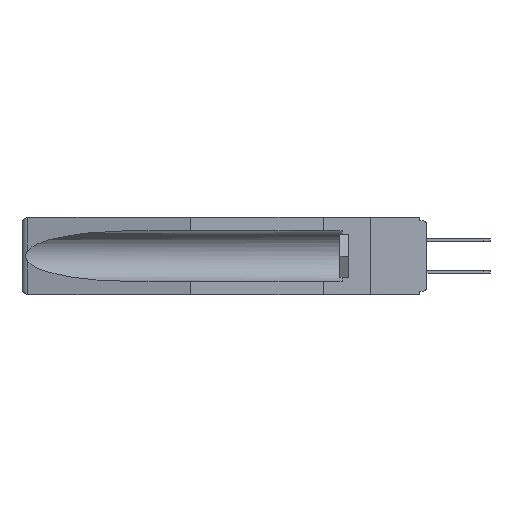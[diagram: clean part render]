
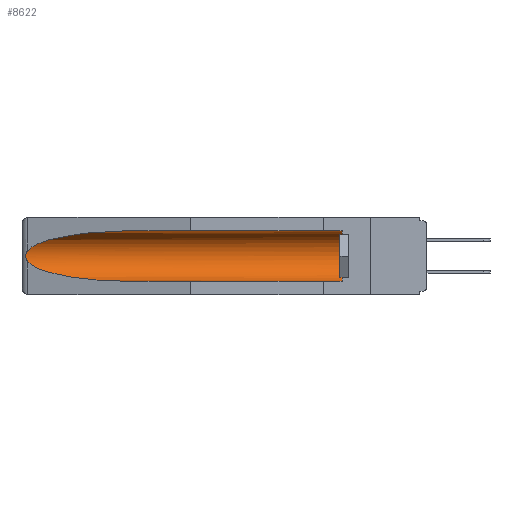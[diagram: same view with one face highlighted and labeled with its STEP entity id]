
A CAD part, left-side view. The second image highlights one B-rep face of the part: STEP entity #8622.
In plain terms, the highlighted cylindrical face has radius 2.857 mm (diameter 5.715 mm), a partial arc.
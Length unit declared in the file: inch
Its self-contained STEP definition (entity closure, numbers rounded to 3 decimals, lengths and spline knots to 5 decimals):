
#264 = CARTESIAN_POINT ( 'NONE',  ( 0.26537, 1.52718, -0.19328 ) ) ;
#686 = CARTESIAN_POINT ( 'NONE',  ( 0.155, 1.07973, -0.059 ) ) ;
#1372 = VECTOR ( 'NONE', #3937, 39.37008 ) ;
#1509 = CARTESIAN_POINT ( 'NONE',  ( 0.26654, 1.53092, -0.15636 ) ) ;
#1808 = DIRECTION ( 'NONE',  ( 0., -1., 0. ) ) ;
#2744 = CARTESIAN_POINT ( 'NONE',  ( 0.21114, 1.30732, -0.059 ) ) ;
#3155 = CARTESIAN_POINT ( 'NONE',  ( 0.155, 0.126, -0.284 ) ) ;
#3727 = B_SPLINE_CURVE_WITH_KNOTS ( 'NONE', 3,
 ( #22746, #17773, #1509, #5532, #17923, #7298, #10869, #16222, #19556, #264 ),
 .UNSPECIFIED., .F., .F.,
 ( 4, 2, 2, 2, 4 ),
 ( 0., 0.00029, 0.00058, 0.00087, 0.00117 ),
 .UNSPECIFIED. ) ;
#3937 = DIRECTION ( 'NONE',  ( 0., 1., 0. ) ) ;
#4163 = LINE ( 'NONE', #5238, #1372 ) ;
#4314 = CARTESIAN_POINT ( 'NONE',  ( 0.26537, 1.52718, -0.19328 ) ) ;
#5137 = VERTEX_POINT ( 'NONE', #3155 ) ;
#5238 = CARTESIAN_POINT ( 'NONE',  ( 0.155, -0.30754, -0.059 ) ) ;
#5261 = CYLINDRICAL_SURFACE ( 'NONE', #6894, 0.1125 ) ;
#5532 = CARTESIAN_POINT ( 'NONE',  ( 0.2673, 1.5327, -0.16383 ) ) ;
#5998 = EDGE_CURVE ( 'NONE', #5137, #9668, #10401, .T. ) ;
#6894 = AXIS2_PLACEMENT_3D ( 'NONE', #11008, #7442, #7355 ) ;
#7261 = EDGE_CURVE ( 'NONE', #18833, #18517, #3727, .T. ) ;
#7298 = CARTESIAN_POINT ( 'NONE',  ( 0.2675, 1.53308, -0.17534 ) ) ;
#7355 = DIRECTION ( 'NONE',  ( 0., 0., 1. ) ) ;
#7442 = DIRECTION ( 'NONE',  ( 0., 1., 0. ) ) ;
#7665 = ORIENTED_EDGE ( 'NONE', *, *, #5998, .T. ) ;
#7708 = CARTESIAN_POINT ( 'NONE',  ( 0.155, -0.30754, -0.284 ) ) ;
#8604 = AXIS2_PLACEMENT_3D ( 'NONE', #21230, #1808, #14182 ) ;
#8622 = ADVANCED_FACE ( 'NONE', ( #19129 ), #5261, .F. ) ;
#9254 = EDGE_CURVE ( 'NONE', #5137, #14358, #18828, .T. ) ;
#9668 = VERTEX_POINT ( 'NONE', #16982 ) ;
#9707 = CARTESIAN_POINT ( 'NONE',  ( 0.21114, 1.30732, -0.284 ) ) ;
#9817 = EDGE_CURVE ( 'NONE', #9668, #14935, #4163, .T. ) ;
#10401 = CIRCLE ( 'NONE', #8604, 0.1125 ) ;
#10404 = EDGE_LOOP ( 'NONE', ( #12081, #18939, #14210, #19327, #7665, #17297 ) ) ;
#10869 = CARTESIAN_POINT ( 'NONE',  ( 0.2673, 1.53269, -0.17917 ) ) ;
#11008 = CARTESIAN_POINT ( 'NONE',  ( 0.155, -0.30754, -0.1715 ) ) ;
#12062 = CARTESIAN_POINT ( 'NONE',  ( 0.25451, 1.48313, -0.09465 ) ) ;
#12081 = ORIENTED_EDGE ( 'NONE', *, *, #14480, .T. ) ;
#12601 = CARTESIAN_POINT ( 'NONE',  ( 0.26537, 1.52718, -0.14972 ) ) ;
#12926 =( BOUNDED_CURVE ( )  B_SPLINE_CURVE ( 3, ( #4314, #18475, #9707, #22107 ),
 .UNSPECIFIED., .F., .F. ) 
 B_SPLINE_CURVE_WITH_KNOTS ( ( 4, 4 ),
 ( 0.1948, 1.5708 ),
 .UNSPECIFIED. ) 
 CURVE ( )  GEOMETRIC_REPRESENTATION_ITEM ( )  RATIONAL_B_SPLINE_CURVE ( ( 1., 0.848, 0.848, 1. ) ) 
 REPRESENTATION_ITEM ( '' )  );
#13248 = CARTESIAN_POINT ( 'NONE',  ( 0.155, 1.07973, -0.059 ) ) ;
#13639 =( BOUNDED_CURVE ( )  B_SPLINE_CURVE ( 3, ( #13248, #2744, #12062, #13708 ),
 .UNSPECIFIED., .F., .F. ) 
 B_SPLINE_CURVE_WITH_KNOTS ( ( 4, 4 ),
 ( 4.71239, 6.08839 ),
 .UNSPECIFIED. ) 
 CURVE ( )  GEOMETRIC_REPRESENTATION_ITEM ( )  RATIONAL_B_SPLINE_CURVE ( ( 1., 0.848, 0.848, 1. ) ) 
 REPRESENTATION_ITEM ( '' )  );
#13708 = CARTESIAN_POINT ( 'NONE',  ( 0.26537, 1.52718, -0.14972 ) ) ;
#14182 = DIRECTION ( 'NONE',  ( 0., 0., 1. ) ) ;
#14210 = ORIENTED_EDGE ( 'NONE', *, *, #22087, .T. ) ;
#14358 = VERTEX_POINT ( 'NONE', #20689 ) ;
#14480 = EDGE_CURVE ( 'NONE', #14935, #18833, #13639, .T. ) ;
#14935 = VERTEX_POINT ( 'NONE', #686 ) ;
#16222 = CARTESIAN_POINT ( 'NONE',  ( 0.26655, 1.53094, -0.18657 ) ) ;
#16982 = CARTESIAN_POINT ( 'NONE',  ( 0.155, 0.126, -0.059 ) ) ;
#17297 = ORIENTED_EDGE ( 'NONE', *, *, #9817, .T. ) ;
#17773 = CARTESIAN_POINT ( 'NONE',  ( 0.26597, 1.52961, -0.15275 ) ) ;
#17923 = CARTESIAN_POINT ( 'NONE',  ( 0.2675, 1.53308, -0.16763 ) ) ;
#18475 = CARTESIAN_POINT ( 'NONE',  ( 0.25451, 1.48313, -0.24835 ) ) ;
#18517 = VERTEX_POINT ( 'NONE', #22250 ) ;
#18828 = LINE ( 'NONE', #7708, #20516 ) ;
#18833 = VERTEX_POINT ( 'NONE', #12601 ) ;
#18939 = ORIENTED_EDGE ( 'NONE', *, *, #7261, .T. ) ;
#19129 = FACE_OUTER_BOUND ( 'NONE', #10404, .T. ) ;
#19327 = ORIENTED_EDGE ( 'NONE', *, *, #9254, .F. ) ;
#19556 = CARTESIAN_POINT ( 'NONE',  ( 0.26597, 1.5296, -0.19026 ) ) ;
#20021 = DIRECTION ( 'NONE',  ( 0., 1., 0. ) ) ;
#20516 = VECTOR ( 'NONE', #20021, 39.37008 ) ;
#20689 = CARTESIAN_POINT ( 'NONE',  ( 0.155, 1.07973, -0.284 ) ) ;
#21230 = CARTESIAN_POINT ( 'NONE',  ( 0.155, 0.126, -0.1715 ) ) ;
#22087 = EDGE_CURVE ( 'NONE', #18517, #14358, #12926, .T. ) ;
#22107 = CARTESIAN_POINT ( 'NONE',  ( 0.155, 1.07973, -0.284 ) ) ;
#22250 = CARTESIAN_POINT ( 'NONE',  ( 0.26537, 1.52718, -0.19328 ) ) ;
#22746 = CARTESIAN_POINT ( 'NONE',  ( 0.26537, 1.52718, -0.14972 ) ) ;
